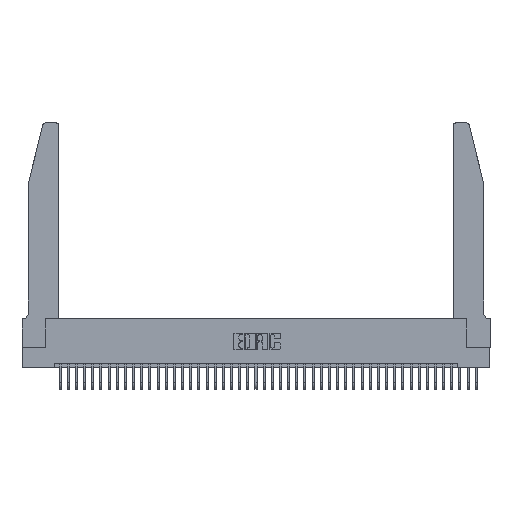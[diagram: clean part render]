
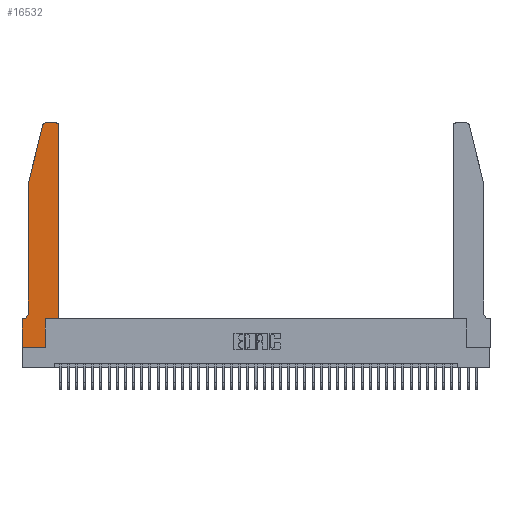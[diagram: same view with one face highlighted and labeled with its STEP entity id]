
A CAD part, top view. The second image highlights one B-rep face of the part: STEP entity #16532.
In plain terms, the highlighted planar face has unit normal (0, 0, 1).
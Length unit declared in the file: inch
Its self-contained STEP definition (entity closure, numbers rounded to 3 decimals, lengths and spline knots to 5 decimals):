
#44 = CARTESIAN_POINT ( 'NONE',  ( 0.0055, 0.35, 0.37 ) ) ;
#95 = VERTEX_POINT ( 'NONE', #25036 ) ;
#436 = CARTESIAN_POINT ( 'NONE',  ( 0.0755, 2., 0.37 ) ) ;
#686 = VECTOR ( 'NONE', #18946, 39.37008 ) ;
#758 = EDGE_CURVE ( 'NONE', #95, #12377, #12718, .T. ) ;
#1562 = CARTESIAN_POINT ( 'NONE',  ( 0.4205, 2.72, 0.37 ) ) ;
#1712 = VECTOR ( 'NONE', #15782, 39.37008 ) ;
#1763 = AXIS2_PLACEMENT_3D ( 'NONE', #29145, #10316, #32256 ) ;
#2953 = CARTESIAN_POINT ( 'NONE',  ( 0., 0., 0.37 ) ) ;
#2983 = ORIENTED_EDGE ( 'NONE', *, *, #39227, .T. ) ;
#3017 = CARTESIAN_POINT ( 'NONE',  ( 0.4505, 0.35, 0.37 ) ) ;
#3268 = ORIENTED_EDGE ( 'NONE', *, *, #3579, .T. ) ;
#3579 = EDGE_CURVE ( 'NONE', #12377, #10350, #23396, .T. ) ;
#3634 = VERTEX_POINT ( 'NONE', #17920 ) ;
#3693 = VECTOR ( 'NONE', #28583, 39.37008 ) ;
#3707 = CARTESIAN_POINT ( 'NONE',  ( 0.2865, 0.35, 0.37 ) ) ;
#4774 = DIRECTION ( 'NONE',  ( 1., 0., 0. ) ) ;
#6096 = CARTESIAN_POINT ( 'NONE',  ( 0.2865, 0.35, 0.37 ) ) ;
#6958 = DIRECTION ( 'NONE',  ( 0., 1., 0. ) ) ;
#8666 = VECTOR ( 'NONE', #12639, 39.37008 ) ;
#9713 = VECTOR ( 'NONE', #13440, 39.37008 ) ;
#9961 = EDGE_CURVE ( 'NONE', #39371, #30705, #38215, .T. ) ;
#9994 = VECTOR ( 'NONE', #32402, 39.37008 ) ;
#10316 = DIRECTION ( 'NONE',  ( 0., 0., 1. ) ) ;
#10350 = VERTEX_POINT ( 'NONE', #33637 ) ;
#10658 = VECTOR ( 'NONE', #6958, 39.37008 ) ;
#10789 = CARTESIAN_POINT ( 'NONE',  ( 0., 0., 0.37 ) ) ;
#11323 = AXIS2_PLACEMENT_3D ( 'NONE', #1562, #23844, #4774 ) ;
#11355 = CARTESIAN_POINT ( 'NONE',  ( 0.284, 2.72, 0.37 ) ) ;
#12377 = VERTEX_POINT ( 'NONE', #28320 ) ;
#12454 = ORIENTED_EDGE ( 'NONE', *, *, #758, .T. ) ;
#12639 = DIRECTION ( 'NONE',  ( -0.239, -0.971, 0. ) ) ;
#12661 = ORIENTED_EDGE ( 'NONE', *, *, #26348, .T. ) ;
#12718 = LINE ( 'NONE', #23185, #36633 ) ;
#12744 = CARTESIAN_POINT ( 'NONE',  ( 0.0755, 2., 0.37 ) ) ;
#12751 = ORIENTED_EDGE ( 'NONE', *, *, #30452, .T. ) ;
#13008 = VERTEX_POINT ( 'NONE', #6096 ) ;
#13440 = DIRECTION ( 'NONE',  ( 0., -1., 0. ) ) ;
#14151 = CARTESIAN_POINT ( 'NONE',  ( 0.4505, 2.72, 0.37 ) ) ;
#14605 = DIRECTION ( 'NONE',  ( 1., 0., 0. ) ) ;
#15328 = ORIENTED_EDGE ( 'NONE', *, *, #21863, .T. ) ;
#15782 = DIRECTION ( 'NONE',  ( 0., -1., 0. ) ) ;
#16532 = ADVANCED_FACE ( 'NONE', ( #28331 ), #19775, .T. ) ;
#17199 = LINE ( 'NONE', #21993, #8666 ) ;
#17805 = LINE ( 'NONE', #34426, #1712 ) ;
#17920 = CARTESIAN_POINT ( 'NONE',  ( 0.0755, 0.42, 0.37 ) ) ;
#18026 = VERTEX_POINT ( 'NONE', #21818 ) ;
#18105 = VERTEX_POINT ( 'NONE', #12744 ) ;
#18189 = DIRECTION ( 'NONE',  ( 0., 0., -1. ) ) ;
#18199 = LINE ( 'NONE', #436, #9713 ) ;
#18946 = DIRECTION ( 'NONE',  ( 0., 1., 0. ) ) ;
#19775 = PLANE ( 'NONE',  #1763 ) ;
#20432 = ORIENTED_EDGE ( 'NONE', *, *, #38220, .T. ) ;
#21818 = CARTESIAN_POINT ( 'NONE',  ( 0., 0.35, 0.37 ) ) ;
#21863 = EDGE_CURVE ( 'NONE', #18105, #3634, #18199, .T. ) ;
#21993 = CARTESIAN_POINT ( 'NONE',  ( 0.0755, 2., 0.37 ) ) ;
#22906 = CIRCLE ( 'NONE', #39648, 0.07 ) ;
#23185 = CARTESIAN_POINT ( 'NONE',  ( 0.2605, 2.75, 0.37 ) ) ;
#23396 = CIRCLE ( 'NONE', #33680, 0.03 ) ;
#23403 = EDGE_CURVE ( 'NONE', #3634, #36537, #22906, .T. ) ;
#23844 = DIRECTION ( 'NONE',  ( 0., 0., 1. ) ) ;
#23899 = VERTEX_POINT ( 'NONE', #14151 ) ;
#24187 = EDGE_CURVE ( 'NONE', #13008, #25278, #35019, .T. ) ;
#24684 = ORIENTED_EDGE ( 'NONE', *, *, #24187, .T. ) ;
#25036 = CARTESIAN_POINT ( 'NONE',  ( 0.4205, 2.75, 0.37 ) ) ;
#25050 = CARTESIAN_POINT ( 'NONE',  ( 0.4505, 0.35, 0.37 ) ) ;
#25278 = VERTEX_POINT ( 'NONE', #3017 ) ;
#26049 = LINE ( 'NONE', #25050, #686 ) ;
#26147 = CARTESIAN_POINT ( 'NONE',  ( 0.2865, 0., 0.37 ) ) ;
#26338 = EDGE_CURVE ( 'NONE', #18026, #39371, #17805, .T. ) ;
#26348 = EDGE_CURVE ( 'NONE', #25278, #23899, #26049, .T. ) ;
#26456 = CIRCLE ( 'NONE', #11323, 0.03 ) ;
#26821 = ORIENTED_EDGE ( 'NONE', *, *, #26338, .T. ) ;
#26889 = ORIENTED_EDGE ( 'NONE', *, *, #23403, .T. ) ;
#27714 = VECTOR ( 'NONE', #28215, 39.37008 ) ;
#28215 = DIRECTION ( 'NONE',  ( -1., 0., 0. ) ) ;
#28320 = CARTESIAN_POINT ( 'NONE',  ( 0.284, 2.75, 0.37 ) ) ;
#28331 = FACE_OUTER_BOUND ( 'NONE', #31914, .T. ) ;
#28583 = DIRECTION ( 'NONE',  ( 1., 0., 0. ) ) ;
#29145 = CARTESIAN_POINT ( 'NONE',  ( 0., 0.35, 0.37 ) ) ;
#29282 = CARTESIAN_POINT ( 'NONE',  ( 0.4505, 0.35, 0.37 ) ) ;
#29610 = ORIENTED_EDGE ( 'NONE', *, *, #9961, .T. ) ;
#30372 = ORIENTED_EDGE ( 'NONE', *, *, #33648, .T. ) ;
#30452 = EDGE_CURVE ( 'NONE', #36537, #18026, #36945, .T. ) ;
#30705 = VERTEX_POINT ( 'NONE', #26147 ) ;
#31914 = EDGE_LOOP ( 'NONE', ( #12454, #3268, #20432, #15328, #26889, #12751, #26821, #29610, #2983, #24684, #12661, #30372 ) ) ;
#32256 = DIRECTION ( 'NONE',  ( 1., 0., 0. ) ) ;
#32402 = DIRECTION ( 'NONE',  ( 1., 0., 0. ) ) ;
#33280 = DIRECTION ( 'NONE',  ( 0., 0., 1. ) ) ;
#33637 = CARTESIAN_POINT ( 'NONE',  ( 0.25487, 2.72718, 0.37 ) ) ;
#33648 = EDGE_CURVE ( 'NONE', #23899, #95, #26456, .T. ) ;
#33680 = AXIS2_PLACEMENT_3D ( 'NONE', #11355, #33280, #14605 ) ;
#34426 = CARTESIAN_POINT ( 'NONE',  ( 0., 0., 0.37 ) ) ;
#35019 = LINE ( 'NONE', #29282, #9994 ) ;
#35170 = DIRECTION ( 'NONE',  ( -1., 0., 0. ) ) ;
#36537 = VERTEX_POINT ( 'NONE', #44 ) ;
#36624 = LINE ( 'NONE', #3707, #10658 ) ;
#36633 = VECTOR ( 'NONE', #35170, 39.37008 ) ;
#36791 = CARTESIAN_POINT ( 'NONE',  ( 0.0055, 0.42, 0.37 ) ) ;
#36945 = LINE ( 'NONE', #37464, #27714 ) ;
#37464 = CARTESIAN_POINT ( 'NONE',  ( 0.0755, 0.35, 0.37 ) ) ;
#38215 = LINE ( 'NONE', #2953, #3693 ) ;
#38220 = EDGE_CURVE ( 'NONE', #10350, #18105, #17199, .T. ) ;
#39227 = EDGE_CURVE ( 'NONE', #30705, #13008, #36624, .T. ) ;
#39371 = VERTEX_POINT ( 'NONE', #10789 ) ;
#39648 = AXIS2_PLACEMENT_3D ( 'NONE', #36791, #18189, #39900 ) ;
#39900 = DIRECTION ( 'NONE',  ( -1., 0., 0. ) ) ;
